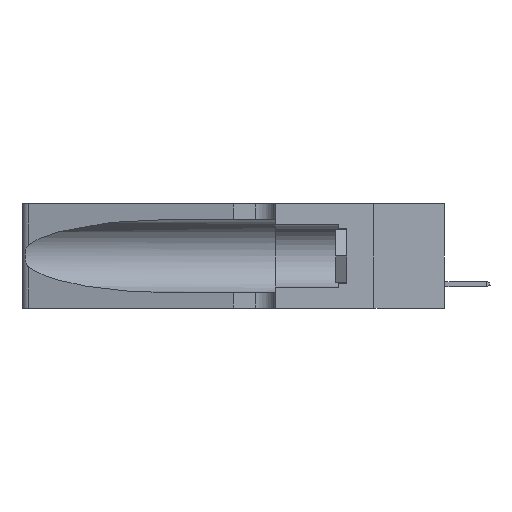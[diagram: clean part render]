
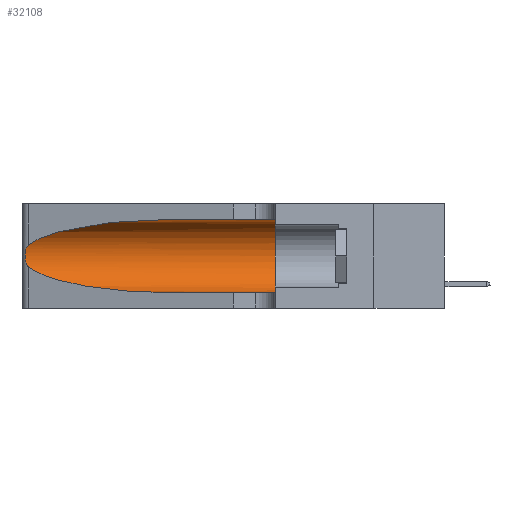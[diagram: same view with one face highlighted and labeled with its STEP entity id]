
A CAD part, left-side view. The second image highlights one B-rep face of the part: STEP entity #32108.
In plain terms, the highlighted cylindrical face has radius 3.308 mm (diameter 6.617 mm), a partial arc.
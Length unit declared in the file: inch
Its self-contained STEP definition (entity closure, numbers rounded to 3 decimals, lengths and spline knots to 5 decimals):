
#84 = CARTESIAN_POINT ( 'NONE',  ( 0.1305, 1.61858, 0.185 ) ) ;
#579 = ORIENTED_EDGE ( 'NONE', *, *, #2225, .T. ) ;
#1248 = EDGE_LOOP ( 'NONE', ( #579, #12139, #21729, #45234, #42631, #8730 ) ) ;
#2225 = EDGE_CURVE ( 'NONE', #47113, #17430, #9017, .T. ) ;
#2700 = CARTESIAN_POINT ( 'NONE',  ( 0.26075, 1.23896, 0.178 ) ) ;
#3022 = CARTESIAN_POINT ( 'NONE',  ( 0.25787, 1.23484, 0.2124 ) ) ;
#3474 = CARTESIAN_POINT ( 'NONE',  ( 0.25487, 1.22718, 0.22369 ) ) ;
#5309 = CARTESIAN_POINT ( 'NONE',  ( 0.1305, 0.72297, 0.05475 ) ) ;
#6956 = CYLINDRICAL_SURFACE ( 'NONE', #43070, 0.13025 ) ;
#8702 = CARTESIAN_POINT ( 'NONE',  ( 0.1305, 1.61858, 0.31525 ) ) ;
#8730 = ORIENTED_EDGE ( 'NONE', *, *, #31740, .F. ) ;
#9017 =( BOUNDED_CURVE ( )  B_SPLINE_CURVE ( 3, ( #28086, #21017, #46630, #24692 ),
 .UNSPECIFIED., .F., .T. ) 
 B_SPLINE_CURVE_WITH_KNOTS ( ( 4, 4 ),
 ( 1.5708, 2.84003 ),
 .UNSPECIFIED. ) 
 CURVE ( )  GEOMETRIC_REPRESENTATION_ITEM ( )  RATIONAL_B_SPLINE_CURVE ( ( 1., 0.87, 0.87, 1. ) ) 
 REPRESENTATION_ITEM ( '' )  );
#9598 = CARTESIAN_POINT ( 'NONE',  ( 0.25487, 1.22718, 0.14631 ) ) ;
#9894 = CARTESIAN_POINT ( 'NONE',  ( 0.26017, 1.23833, 0.17102 ) ) ;
#10245 = EDGE_CURVE ( 'NONE', #17430, #28992, #23069, .T. ) ;
#11111 = DIRECTION ( 'NONE',  ( 0., 0., 1. ) ) ;
#11278 = CARTESIAN_POINT ( 'NONE',  ( 0.1305, 0.72297, 0.05475 ) ) ;
#11484 = CIRCLE ( 'NONE', #37611, 0.13025 ) ;
#11867 = CARTESIAN_POINT ( 'NONE',  ( 0.25487, 1.22718, 0.14631 ) ) ;
#12139 = ORIENTED_EDGE ( 'NONE', *, *, #10245, .T. ) ;
#12824 = LINE ( 'NONE', #41652, #24923 ) ;
#17255 = CARTESIAN_POINT ( 'NONE',  ( 0.25856, 1.23593, 0.16098 ) ) ;
#17430 = VERTEX_POINT ( 'NONE', #3474 ) ;
#17563 = CARTESIAN_POINT ( 'NONE',  ( 0.26075, 1.23896, 0.19203 ) ) ;
#18477 = CARTESIAN_POINT ( 'NONE',  ( 0.18966, 0.96281, 0.05475 ) ) ;
#21017 = CARTESIAN_POINT ( 'NONE',  ( 0.18966, 0.96281, 0.31525 ) ) ;
#21729 = ORIENTED_EDGE ( 'NONE', *, *, #23770, .T. ) ;
#22017 = DIRECTION ( 'NONE',  ( 0., 0., -1. ) ) ;
#23069 = B_SPLINE_CURVE_WITH_KNOTS ( 'NONE', 3,
 ( #39062, #46411, #24801, #3022, #24481, #28191, #17563, #2700, #9894, #17255, #42905, #32184, #28343, #35706 ),
 .UNSPECIFIED., .F., .F.,
 ( 4, 2, 2, 2, 2, 2, 4 ),
 ( 0., 0.00027, 0.00053, 0.00107, 0.0016, 0.00187, 0.00214 ),
 .UNSPECIFIED. ) ;
#23770 = EDGE_CURVE ( 'NONE', #28992, #34181, #35221, .T. ) ;
#23802 = CARTESIAN_POINT ( 'NONE',  ( 0.1305, 0.35, 0.31525 ) ) ;
#24481 = CARTESIAN_POINT ( 'NONE',  ( 0.25854, 1.2359, 0.20912 ) ) ;
#24692 = CARTESIAN_POINT ( 'NONE',  ( 0.25487, 1.22718, 0.22369 ) ) ;
#24801 = CARTESIAN_POINT ( 'NONE',  ( 0.25639, 1.23184, 0.21858 ) ) ;
#24923 = VECTOR ( 'NONE', #31284, 39.37008 ) ;
#26155 = VERTEX_POINT ( 'NONE', #23802 ) ;
#27040 = LINE ( 'NONE', #8702, #36796 ) ;
#28086 = CARTESIAN_POINT ( 'NONE',  ( 0.1305, 0.72297, 0.31525 ) ) ;
#28191 = CARTESIAN_POINT ( 'NONE',  ( 0.26018, 1.23835, 0.19895 ) ) ;
#28343 = CARTESIAN_POINT ( 'NONE',  ( 0.25555, 1.22993, 0.14849 ) ) ;
#28992 = VERTEX_POINT ( 'NONE', #9598 ) ;
#30944 = DIRECTION ( 'NONE',  ( 0., -1., 0. ) ) ;
#31052 = FACE_OUTER_BOUND ( 'NONE', #1248, .T. ) ;
#31284 = DIRECTION ( 'NONE',  ( 0., -1., 0. ) ) ;
#31740 = EDGE_CURVE ( 'NONE', #47113, #26155, #27040, .T. ) ;
#32108 = ADVANCED_FACE ( 'NONE', ( #31052 ), #6956, .F. ) ;
#32184 = CARTESIAN_POINT ( 'NONE',  ( 0.25639, 1.23186, 0.15144 ) ) ;
#33351 = CARTESIAN_POINT ( 'NONE',  ( 0.1305, 0.35, 0.185 ) ) ;
#34181 = VERTEX_POINT ( 'NONE', #11278 ) ;
#34227 = VERTEX_POINT ( 'NONE', #34297 ) ;
#34297 = CARTESIAN_POINT ( 'NONE',  ( 0.1305, 0.35, 0.05475 ) ) ;
#35221 =( BOUNDED_CURVE ( )  B_SPLINE_CURVE ( 3, ( #11867, #40706, #18477, #5309 ),
 .UNSPECIFIED., .F., .T. ) 
 B_SPLINE_CURVE_WITH_KNOTS ( ( 4, 4 ),
 ( 3.44316, 4.71239 ),
 .UNSPECIFIED. ) 
 CURVE ( )  GEOMETRIC_REPRESENTATION_ITEM ( )  RATIONAL_B_SPLINE_CURVE ( ( 1., 0.87, 0.87, 1. ) ) 
 REPRESENTATION_ITEM ( '' )  );
#35706 = CARTESIAN_POINT ( 'NONE',  ( 0.25487, 1.22718, 0.14631 ) ) ;
#36740 = DIRECTION ( 'NONE',  ( 0., 1., 0. ) ) ;
#36796 = VECTOR ( 'NONE', #38341, 39.37008 ) ;
#37122 = CARTESIAN_POINT ( 'NONE',  ( 0.1305, 0.72297, 0.31525 ) ) ;
#37218 = EDGE_CURVE ( 'NONE', #26155, #34227, #11484, .T. ) ;
#37611 = AXIS2_PLACEMENT_3D ( 'NONE', #33351, #36740, #11111 ) ;
#38341 = DIRECTION ( 'NONE',  ( 0., -1., 0. ) ) ;
#39062 = CARTESIAN_POINT ( 'NONE',  ( 0.25487, 1.22718, 0.22369 ) ) ;
#40706 = CARTESIAN_POINT ( 'NONE',  ( 0.2373, 1.15595, 0.08982 ) ) ;
#40994 = EDGE_CURVE ( 'NONE', #34181, #34227, #12824, .T. ) ;
#41652 = CARTESIAN_POINT ( 'NONE',  ( 0.1305, 1.61858, 0.05475 ) ) ;
#42631 = ORIENTED_EDGE ( 'NONE', *, *, #37218, .F. ) ;
#42905 = CARTESIAN_POINT ( 'NONE',  ( 0.25789, 1.23486, 0.15765 ) ) ;
#43070 = AXIS2_PLACEMENT_3D ( 'NONE', #84, #30944, #22017 ) ;
#45234 = ORIENTED_EDGE ( 'NONE', *, *, #40994, .T. ) ;
#46411 = CARTESIAN_POINT ( 'NONE',  ( 0.25555, 1.22994, 0.2215 ) ) ;
#46630 = CARTESIAN_POINT ( 'NONE',  ( 0.2373, 1.15595, 0.28018 ) ) ;
#47113 = VERTEX_POINT ( 'NONE', #37122 ) ;
